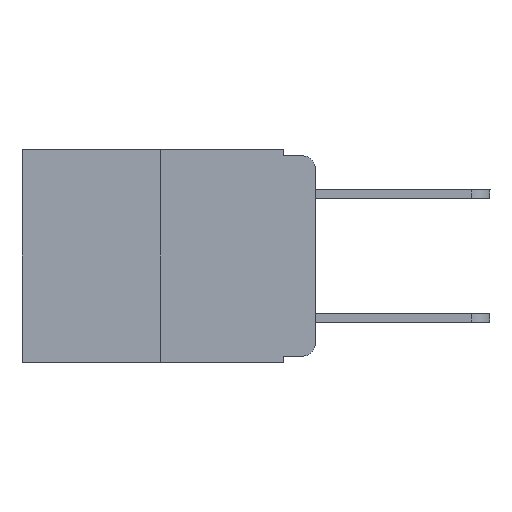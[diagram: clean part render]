
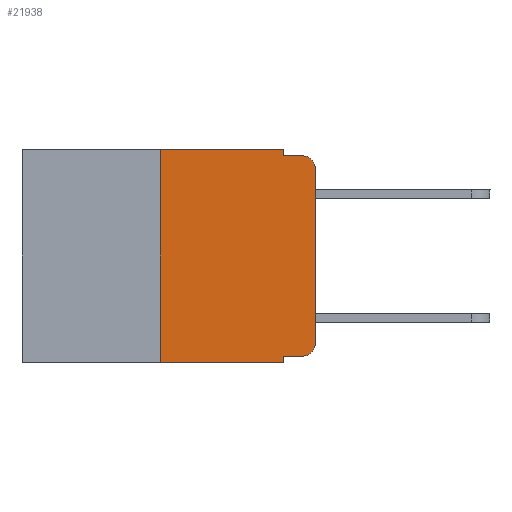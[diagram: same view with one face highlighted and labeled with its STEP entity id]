
A CAD part, left-side view. The second image highlights one B-rep face of the part: STEP entity #21938.
In plain terms, the highlighted planar face has unit normal (-1, 0, 0).
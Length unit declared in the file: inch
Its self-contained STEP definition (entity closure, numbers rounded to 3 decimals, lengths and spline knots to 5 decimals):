
#2 = VERTEX_POINT ( 'NONE', #20787 ) ;
#25 = CARTESIAN_POINT ( 'NONE',  ( 0., 0.051, -0.333 ) ) ;
#33 = LINE ( 'NONE', #12828, #4668 ) ;
#167 = CARTESIAN_POINT ( 'NONE',  ( 0., 0.051, 0. ) ) ;
#909 = DIRECTION ( 'NONE',  ( -1., 0., 0. ) ) ;
#1190 = CARTESIAN_POINT ( 'NONE',  ( 0., 0.02, -0.01 ) ) ;
#1250 = VERTEX_POINT ( 'NONE', #25 ) ;
#1552 = EDGE_LOOP ( 'NONE', ( #8824, #4854, #3769, #4064, #15648, #7309, #18988, #2597, #22672, #12910 ) ) ;
#1586 = VECTOR ( 'NONE', #17754, 39.37008 ) ;
#1812 = VERTEX_POINT ( 'NONE', #9452 ) ;
#1914 = AXIS2_PLACEMENT_3D ( 'NONE', #13022, #909, #3176 ) ;
#2000 = EDGE_CURVE ( 'NONE', #14328, #1812, #15943, .T. ) ;
#2597 = ORIENTED_EDGE ( 'NONE', *, *, #3641, .F. ) ;
#2616 = CARTESIAN_POINT ( 'NONE',  ( 0., 0.051, -0.01 ) ) ;
#3176 = DIRECTION ( 'NONE',  ( 0., 0., -1. ) ) ;
#3368 = CARTESIAN_POINT ( 'NONE',  ( 0., 0.02, -0.03 ) ) ;
#3641 = EDGE_CURVE ( 'NONE', #1250, #2, #16823, .T. ) ;
#3769 = ORIENTED_EDGE ( 'NONE', *, *, #17578, .F. ) ;
#3833 = EDGE_CURVE ( 'NONE', #7395, #20572, #4944, .T. ) ;
#4064 = ORIENTED_EDGE ( 'NONE', *, *, #21130, .F. ) ;
#4668 = VECTOR ( 'NONE', #7100, 39.37008 ) ;
#4854 = ORIENTED_EDGE ( 'NONE', *, *, #5536, .T. ) ;
#4944 = LINE ( 'NONE', #11429, #23086 ) ;
#5536 = EDGE_CURVE ( 'NONE', #1812, #11174, #15756, .T. ) ;
#6452 = CARTESIAN_POINT ( 'NONE',  ( 0., 0.473, 0. ) ) ;
#6708 = LINE ( 'NONE', #2616, #9823 ) ;
#6821 = LINE ( 'NONE', #13677, #1586 ) ;
#6972 = CARTESIAN_POINT ( 'NONE',  ( 0., 0.25, 0. ) ) ;
#7041 = VECTOR ( 'NONE', #20337, 39.37008 ) ;
#7100 = DIRECTION ( 'NONE',  ( 0., -1., 0. ) ) ;
#7206 = CARTESIAN_POINT ( 'NONE',  ( 0., 0.051, -0.01 ) ) ;
#7309 = ORIENTED_EDGE ( 'NONE', *, *, #13078, .F. ) ;
#7395 = VERTEX_POINT ( 'NONE', #8307 ) ;
#7959 = DIRECTION ( 'NONE',  ( 0., 0., -1. ) ) ;
#8307 = CARTESIAN_POINT ( 'NONE',  ( 0., 0.25, 0. ) ) ;
#8410 = VECTOR ( 'NONE', #7959, 39.37008 ) ;
#8762 = DIRECTION ( 'NONE',  ( 1., 0., 0. ) ) ;
#8824 = ORIENTED_EDGE ( 'NONE', *, *, #2000, .T. ) ;
#9452 = CARTESIAN_POINT ( 'NONE',  ( 0., 0., -0.03 ) ) ;
#9531 = VERTEX_POINT ( 'NONE', #18167 ) ;
#9800 = DIRECTION ( 'NONE',  ( 0., -1., 0. ) ) ;
#9823 = VECTOR ( 'NONE', #23787, 39.37008 ) ;
#10355 = EDGE_CURVE ( 'NONE', #1250, #9531, #33, .T. ) ;
#11174 = VERTEX_POINT ( 'NONE', #1190 ) ;
#11429 = CARTESIAN_POINT ( 'NONE',  ( 0., 0.473, 0. ) ) ;
#11721 = CARTESIAN_POINT ( 'NONE',  ( 0., 0.051, 0. ) ) ;
#11917 = DIRECTION ( 'NONE',  ( 0., 0., -1. ) ) ;
#12100 = LINE ( 'NONE', #6972, #18875 ) ;
#12365 = DIRECTION ( 'NONE',  ( 0., 0., -1. ) ) ;
#12828 = CARTESIAN_POINT ( 'NONE',  ( 0., 0.051, -0.333 ) ) ;
#12910 = ORIENTED_EDGE ( 'NONE', *, *, #15089, .T. ) ;
#12942 = DIRECTION ( 'NONE',  ( -1., 0., 0. ) ) ;
#13022 = CARTESIAN_POINT ( 'NONE',  ( 0., 0.02, -0.313 ) ) ;
#13078 = EDGE_CURVE ( 'NONE', #22215, #7395, #12100, .T. ) ;
#13677 = CARTESIAN_POINT ( 'NONE',  ( 0., 0.473, -0.343 ) ) ;
#13794 = VERTEX_POINT ( 'NONE', #7206 ) ;
#14328 = VERTEX_POINT ( 'NONE', #24826 ) ;
#15089 = EDGE_CURVE ( 'NONE', #9531, #14328, #17377, .T. ) ;
#15648 = ORIENTED_EDGE ( 'NONE', *, *, #3833, .F. ) ;
#15756 = CIRCLE ( 'NONE', #20161, 0.02 ) ;
#15943 = LINE ( 'NONE', #24056, #7041 ) ;
#16482 = VECTOR ( 'NONE', #11917, 39.37008 ) ;
#16823 = LINE ( 'NONE', #23885, #16482 ) ;
#17012 = FACE_OUTER_BOUND ( 'NONE', #1552, .T. ) ;
#17309 = CARTESIAN_POINT ( 'NONE',  ( 0., 0.25, -0.343 ) ) ;
#17377 = CIRCLE ( 'NONE', #1914, 0.02 ) ;
#17578 = EDGE_CURVE ( 'NONE', #13794, #11174, #6708, .T. ) ;
#17754 = DIRECTION ( 'NONE',  ( 0., -1., 0. ) ) ;
#18167 = CARTESIAN_POINT ( 'NONE',  ( 0., 0.02, -0.333 ) ) ;
#18340 = AXIS2_PLACEMENT_3D ( 'NONE', #6452, #8762, #12365 ) ;
#18875 = VECTOR ( 'NONE', #19026, 39.37008 ) ;
#18988 = ORIENTED_EDGE ( 'NONE', *, *, #21615, .T. ) ;
#19026 = DIRECTION ( 'NONE',  ( 0., 0., 1. ) ) ;
#20161 = AXIS2_PLACEMENT_3D ( 'NONE', #3368, #12942, #21222 ) ;
#20337 = DIRECTION ( 'NONE',  ( 0., 0., 1. ) ) ;
#20572 = VERTEX_POINT ( 'NONE', #167 ) ;
#20709 = LINE ( 'NONE', #11721, #8410 ) ;
#20787 = CARTESIAN_POINT ( 'NONE',  ( 0., 0.051, -0.343 ) ) ;
#21130 = EDGE_CURVE ( 'NONE', #20572, #13794, #20709, .T. ) ;
#21222 = DIRECTION ( 'NONE',  ( 0., 0., -1. ) ) ;
#21615 = EDGE_CURVE ( 'NONE', #22215, #2, #6821, .T. ) ;
#21938 = ADVANCED_FACE ( 'NONE', ( #17012 ), #24532, .F. ) ;
#22215 = VERTEX_POINT ( 'NONE', #17309 ) ;
#22672 = ORIENTED_EDGE ( 'NONE', *, *, #10355, .T. ) ;
#23086 = VECTOR ( 'NONE', #9800, 39.37008 ) ;
#23787 = DIRECTION ( 'NONE',  ( 0., -1., 0. ) ) ;
#23885 = CARTESIAN_POINT ( 'NONE',  ( 0., 0.051, 0. ) ) ;
#24056 = CARTESIAN_POINT ( 'NONE',  ( 0., 0., 0. ) ) ;
#24532 = PLANE ( 'NONE',  #18340 ) ;
#24826 = CARTESIAN_POINT ( 'NONE',  ( 0., 0., -0.313 ) ) ;
